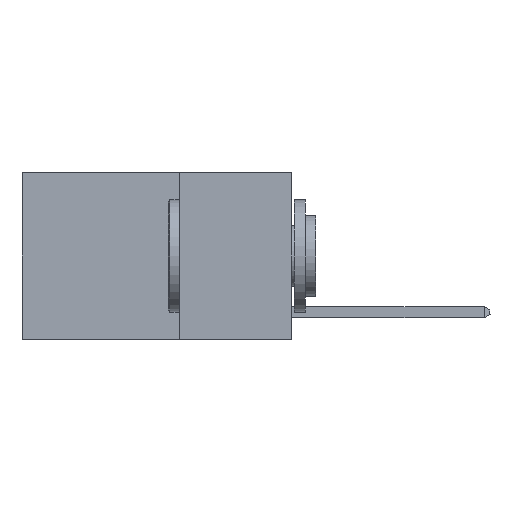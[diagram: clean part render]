
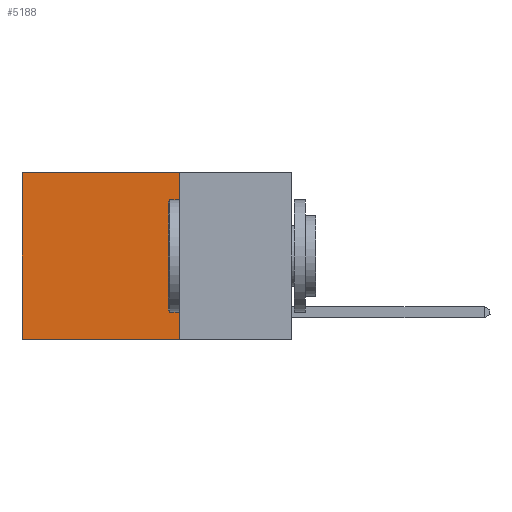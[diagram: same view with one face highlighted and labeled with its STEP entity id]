
A CAD part, left-side view. The second image highlights one B-rep face of the part: STEP entity #5188.
In plain terms, the highlighted planar face has unit normal (-1, 0, 0).
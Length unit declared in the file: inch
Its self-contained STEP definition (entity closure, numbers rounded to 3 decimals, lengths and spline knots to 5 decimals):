
#88 = ORIENTED_EDGE ( 'NONE', *, *, #2704, .F. ) ;
#195 = CARTESIAN_POINT ( 'NONE',  ( 0.2625, 0.25, 0. ) ) ;
#544 = CARTESIAN_POINT ( 'NONE',  ( 0.2625, 0.25, 0. ) ) ;
#569 = VERTEX_POINT ( 'NONE', #2959 ) ;
#624 = PLANE ( 'NONE',  #8892 ) ;
#923 = VECTOR ( 'NONE', #5883, 39.37008 ) ;
#945 = EDGE_LOOP ( 'NONE', ( #5775, #5276, #88, #6846 ) ) ;
#1050 = CARTESIAN_POINT ( 'NONE',  ( 0.2625, 0.6, 0. ) ) ;
#1141 = EDGE_CURVE ( 'NONE', #1437, #569, #7235, .T. ) ;
#1381 = VERTEX_POINT ( 'NONE', #195 ) ;
#1437 = VERTEX_POINT ( 'NONE', #1595 ) ;
#1595 = CARTESIAN_POINT ( 'NONE',  ( 0.2625, 0.25, -0.37 ) ) ;
#2250 = VERTEX_POINT ( 'NONE', #1050 ) ;
#2704 = EDGE_CURVE ( 'NONE', #1381, #1437, #6692, .T. ) ;
#2959 = CARTESIAN_POINT ( 'NONE',  ( 0.2625, 0.6, -0.37 ) ) ;
#4316 = DIRECTION ( 'NONE',  ( 0., 0., -1. ) ) ;
#4443 = LINE ( 'NONE', #8005, #5109 ) ;
#5109 = VECTOR ( 'NONE', #5203, 39.37008 ) ;
#5188 = ADVANCED_FACE ( 'NONE', ( #6836 ), #624, .F. ) ;
#5203 = DIRECTION ( 'NONE',  ( 0., 1., 0. ) ) ;
#5276 = ORIENTED_EDGE ( 'NONE', *, *, #1141, .F. ) ;
#5322 = CARTESIAN_POINT ( 'NONE',  ( 0.2625, 0.6, 0. ) ) ;
#5775 = ORIENTED_EDGE ( 'NONE', *, *, #7564, .T. ) ;
#5883 = DIRECTION ( 'NONE',  ( 0., 1., 0. ) ) ;
#6692 = LINE ( 'NONE', #544, #7345 ) ;
#6836 = FACE_OUTER_BOUND ( 'NONE', #945, .T. ) ;
#6846 = ORIENTED_EDGE ( 'NONE', *, *, #8023, .T. ) ;
#7235 = LINE ( 'NONE', #8669, #923 ) ;
#7345 = VECTOR ( 'NONE', #11241, 39.37008 ) ;
#7564 = EDGE_CURVE ( 'NONE', #2250, #569, #8131, .T. ) ;
#8005 = CARTESIAN_POINT ( 'NONE',  ( 0.2625, 0.25, 0. ) ) ;
#8023 = EDGE_CURVE ( 'NONE', #1381, #2250, #4443, .T. ) ;
#8131 = LINE ( 'NONE', #5322, #9199 ) ;
#8669 = CARTESIAN_POINT ( 'NONE',  ( 0.2625, 0.25, -0.37 ) ) ;
#8787 = DIRECTION ( 'NONE',  ( 1., 0., 0. ) ) ;
#8892 = AXIS2_PLACEMENT_3D ( 'NONE', #11430, #8787, #4316 ) ;
#9199 = VECTOR ( 'NONE', #10802, 39.37008 ) ;
#10802 = DIRECTION ( 'NONE',  ( 0., 0., -1. ) ) ;
#11241 = DIRECTION ( 'NONE',  ( 0., 0., -1. ) ) ;
#11430 = CARTESIAN_POINT ( 'NONE',  ( 0.2625, 0.25, 0. ) ) ;
